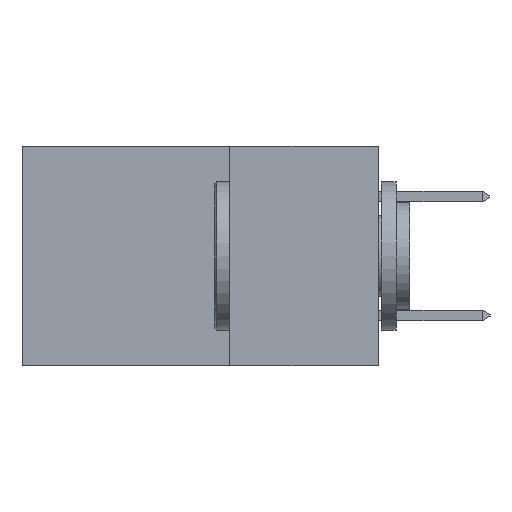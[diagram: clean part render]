
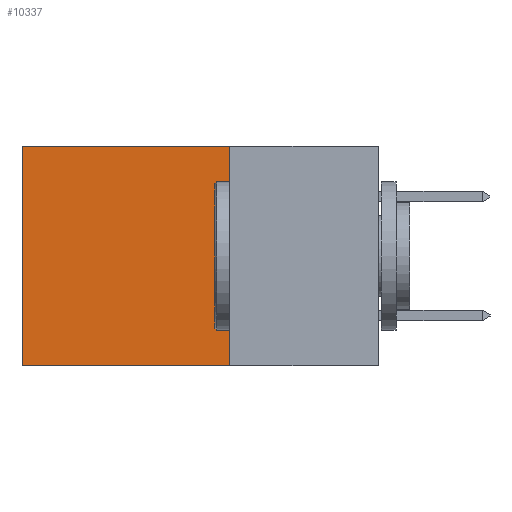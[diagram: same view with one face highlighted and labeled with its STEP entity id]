
A CAD part, left-side view. The second image highlights one B-rep face of the part: STEP entity #10337.
In plain terms, the highlighted planar face has unit normal (-1, 0, 0).
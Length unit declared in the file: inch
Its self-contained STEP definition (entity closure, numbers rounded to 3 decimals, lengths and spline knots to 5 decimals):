
#373 = CARTESIAN_POINT ( 'NONE',  ( 0.2615, 0.25, -0.37 ) ) ;
#1758 = VECTOR ( 'NONE', #7859, 39.37008 ) ;
#1888 = CARTESIAN_POINT ( 'NONE',  ( 0.2615, 0.6, -0.37 ) ) ;
#2212 = DIRECTION ( 'NONE',  ( 0., 0., -1. ) ) ;
#2586 = ORIENTED_EDGE ( 'NONE', *, *, #6395, .F. ) ;
#3616 = CARTESIAN_POINT ( 'NONE',  ( 0.2615, 0.25, 0. ) ) ;
#5891 = CARTESIAN_POINT ( 'NONE',  ( 0.2615, 0.25, -0.37 ) ) ;
#6054 = CARTESIAN_POINT ( 'NONE',  ( 0.2615, 0.25, -0.37 ) ) ;
#6395 = EDGE_CURVE ( 'NONE', #17362, #9833, #10170, .T. ) ;
#7859 = DIRECTION ( 'NONE',  ( 0., 1., 0. ) ) ;
#9099 = DIRECTION ( 'NONE',  ( 0., 0., -1. ) ) ;
#9491 = PLANE ( 'NONE',  #22357 ) ;
#9833 = VERTEX_POINT ( 'NONE', #13420 ) ;
#10170 = LINE ( 'NONE', #373, #18749 ) ;
#10337 = ADVANCED_FACE ( 'NONE', ( #19396 ), #9491, .F. ) ;
#10821 = DIRECTION ( 'NONE',  ( 0., 1., 0. ) ) ;
#11226 = DIRECTION ( 'NONE',  ( 0., 0., -1. ) ) ;
#12212 = ORIENTED_EDGE ( 'NONE', *, *, #16859, .T. ) ;
#13159 = VECTOR ( 'NONE', #9099, 39.37008 ) ;
#13420 = CARTESIAN_POINT ( 'NONE',  ( 0.2615, 0.25, -0.37 ) ) ;
#13535 = EDGE_CURVE ( 'NONE', #17362, #18455, #22653, .T. ) ;
#13549 = VERTEX_POINT ( 'NONE', #1888 ) ;
#13556 = VECTOR ( 'NONE', #10821, 39.37008 ) ;
#14369 = ORIENTED_EDGE ( 'NONE', *, *, #13535, .T. ) ;
#16859 = EDGE_CURVE ( 'NONE', #18455, #13549, #22253, .T. ) ;
#17027 = EDGE_LOOP ( 'NONE', ( #12212, #18416, #2586, #14369 ) ) ;
#17362 = VERTEX_POINT ( 'NONE', #3616 ) ;
#17663 = CARTESIAN_POINT ( 'NONE',  ( 0.2615, 0.25, 0. ) ) ;
#18318 = EDGE_CURVE ( 'NONE', #9833, #13549, #20940, .T. ) ;
#18416 = ORIENTED_EDGE ( 'NONE', *, *, #18318, .F. ) ;
#18455 = VERTEX_POINT ( 'NONE', #20210 ) ;
#18749 = VECTOR ( 'NONE', #2212, 39.37008 ) ;
#19381 = CARTESIAN_POINT ( 'NONE',  ( 0.2615, 0.6, -0.37 ) ) ;
#19396 = FACE_OUTER_BOUND ( 'NONE', #17027, .T. ) ;
#20210 = CARTESIAN_POINT ( 'NONE',  ( 0.2615, 0.6, 0. ) ) ;
#20940 = LINE ( 'NONE', #6054, #1758 ) ;
#21499 = DIRECTION ( 'NONE',  ( 1., 0., 0. ) ) ;
#22253 = LINE ( 'NONE', #19381, #13159 ) ;
#22357 = AXIS2_PLACEMENT_3D ( 'NONE', #5891, #21499, #11226 ) ;
#22653 = LINE ( 'NONE', #17663, #13556 ) ;
